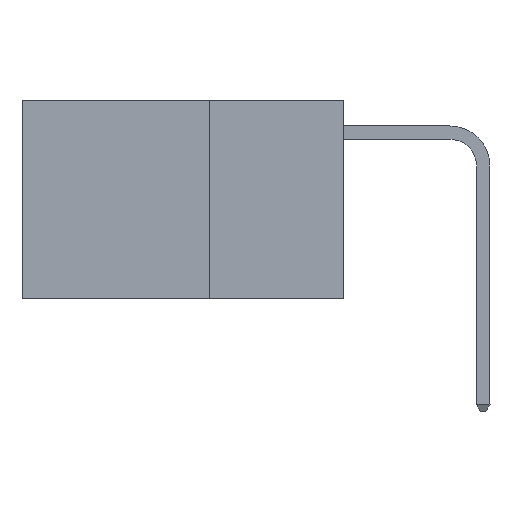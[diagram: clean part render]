
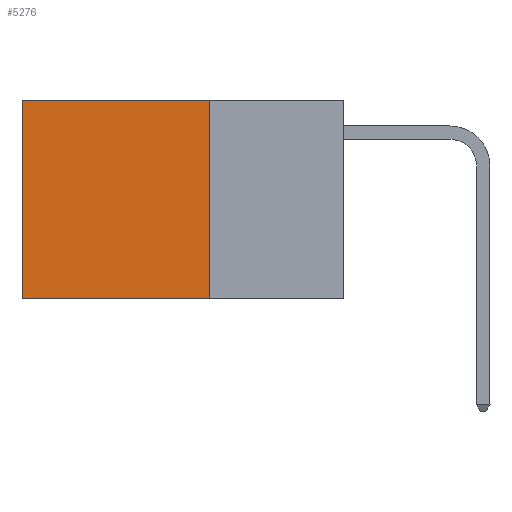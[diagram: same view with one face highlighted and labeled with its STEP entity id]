
A CAD part, left-side view. The second image highlights one B-rep face of the part: STEP entity #5276.
In plain terms, the highlighted planar face has unit normal (-1, 0, 0).
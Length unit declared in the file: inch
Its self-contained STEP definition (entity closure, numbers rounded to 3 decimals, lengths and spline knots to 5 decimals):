
#92 = VERTEX_POINT ( 'NONE', #963 ) ;
#208 = ORIENTED_EDGE ( 'NONE', *, *, #8026, .T. ) ;
#628 = CARTESIAN_POINT ( 'NONE',  ( 0.2625, 0.6, 0. ) ) ;
#775 = EDGE_CURVE ( 'NONE', #10760, #10578, #12133, .T. ) ;
#963 = CARTESIAN_POINT ( 'NONE',  ( 0.2625, 0.6, -0.37 ) ) ;
#990 = VECTOR ( 'NONE', #6915, 39.37008 ) ;
#3030 = DIRECTION ( 'NONE',  ( 0., 1., 0. ) ) ;
#3056 = EDGE_CURVE ( 'NONE', #10760, #11884, #5049, .T. ) ;
#3459 = CARTESIAN_POINT ( 'NONE',  ( 0.2625, 0.6, 0. ) ) ;
#3908 = PLANE ( 'NONE',  #6646 ) ;
#4556 = VECTOR ( 'NONE', #13160, 39.37008 ) ;
#4989 = CARTESIAN_POINT ( 'NONE',  ( 0.2625, 0.25, 0. ) ) ;
#5049 = LINE ( 'NONE', #11549, #7569 ) ;
#5141 = DIRECTION ( 'NONE',  ( 0., 0., -1. ) ) ;
#5276 = ADVANCED_FACE ( 'NONE', ( #7084 ), #3908, .F. ) ;
#5664 = CARTESIAN_POINT ( 'NONE',  ( 0.2625, 0.25, -0.37 ) ) ;
#6646 = AXIS2_PLACEMENT_3D ( 'NONE', #8746, #12415, #5141 ) ;
#6768 = EDGE_LOOP ( 'NONE', ( #208, #9239, #15612, #11398 ) ) ;
#6807 = DIRECTION ( 'NONE',  ( 0., 0., -1. ) ) ;
#6915 = DIRECTION ( 'NONE',  ( 0., 1., 0. ) ) ;
#7084 = FACE_OUTER_BOUND ( 'NONE', #6768, .T. ) ;
#7169 = CARTESIAN_POINT ( 'NONE',  ( 0.2625, 0.25, 0. ) ) ;
#7545 = LINE ( 'NONE', #5664, #990 ) ;
#7569 = VECTOR ( 'NONE', #3030, 39.37008 ) ;
#8026 = EDGE_CURVE ( 'NONE', #11884, #92, #8232, .T. ) ;
#8232 = LINE ( 'NONE', #3459, #4556 ) ;
#8746 = CARTESIAN_POINT ( 'NONE',  ( 0.2625, 0.25, 0. ) ) ;
#8956 = VECTOR ( 'NONE', #6807, 39.37008 ) ;
#9239 = ORIENTED_EDGE ( 'NONE', *, *, #11937, .F. ) ;
#10578 = VERTEX_POINT ( 'NONE', #14909 ) ;
#10760 = VERTEX_POINT ( 'NONE', #7169 ) ;
#11398 = ORIENTED_EDGE ( 'NONE', *, *, #3056, .T. ) ;
#11549 = CARTESIAN_POINT ( 'NONE',  ( 0.2625, 0.25, 0. ) ) ;
#11884 = VERTEX_POINT ( 'NONE', #628 ) ;
#11937 = EDGE_CURVE ( 'NONE', #10578, #92, #7545, .T. ) ;
#12133 = LINE ( 'NONE', #4989, #8956 ) ;
#12415 = DIRECTION ( 'NONE',  ( 1., 0., 0. ) ) ;
#13160 = DIRECTION ( 'NONE',  ( 0., 0., -1. ) ) ;
#14909 = CARTESIAN_POINT ( 'NONE',  ( 0.2625, 0.25, -0.37 ) ) ;
#15612 = ORIENTED_EDGE ( 'NONE', *, *, #775, .F. ) ;
